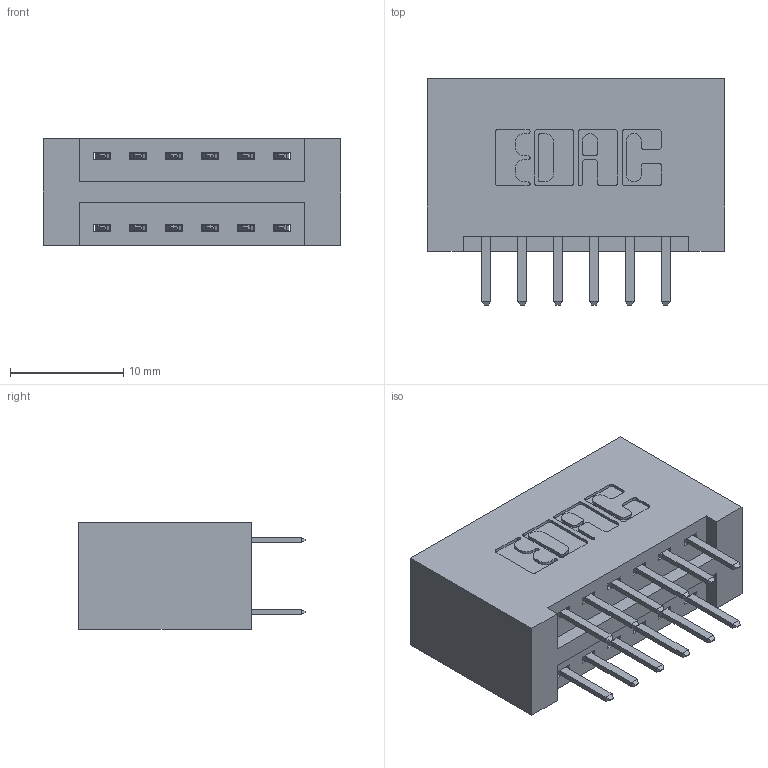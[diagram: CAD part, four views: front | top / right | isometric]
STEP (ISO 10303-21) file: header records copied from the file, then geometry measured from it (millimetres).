
FILE_DESCRIPTION (( 'STEP AP203' ), '1' );
FILE_NAME ('396-012-520-201.STEP', '2019-10-29T19:10:49', ( '' ), ( '' ), 'SwSTEP 2.0', 'SolidWorks 2016', '' );
FILE_SCHEMA (( 'CONFIG_CONTROL_DESIGN' ));
Length unit declared in the file: inch
Products named in the file (3): 396-012-520-201; 345-292-001_345-293-120; 346 Part_No Mounting Lugs
Assembly tree (13 placements, depth 2):
  396-012-520-201
    346 Part_No Mounting Lugs
    345-292-001_345-293-120  x12
Bounding box: 26.29 x 20.02 x 9.4 mm (x, y, z)
Volume: 2851.9 mm3; surface area: 3505.1 mm2
Topology: 13 solids, 13 shells, 786 faces, 2261 edges, 1474 vertices
Faces by surface type: plane 516, cylinder 270
Entity records: 8599 total; most frequent: CARTESIAN_POINT 1476, ORIENTED_EDGE 1398, DIRECTION 1335, EDGE_CURVE 699, LINE 547, VECTOR 547, VERTEX_POINT 462, AXIS2_PLACEMENT_3D 394
